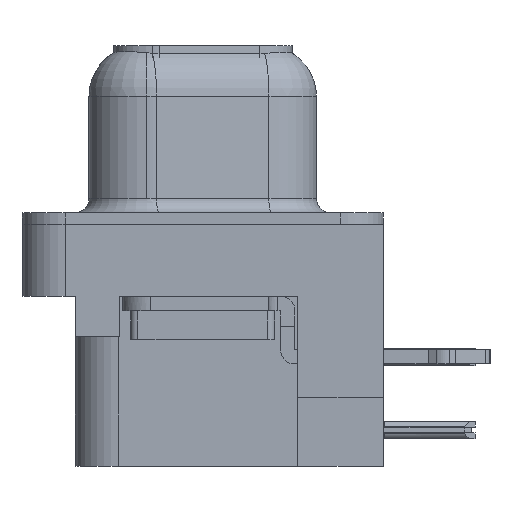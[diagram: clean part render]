
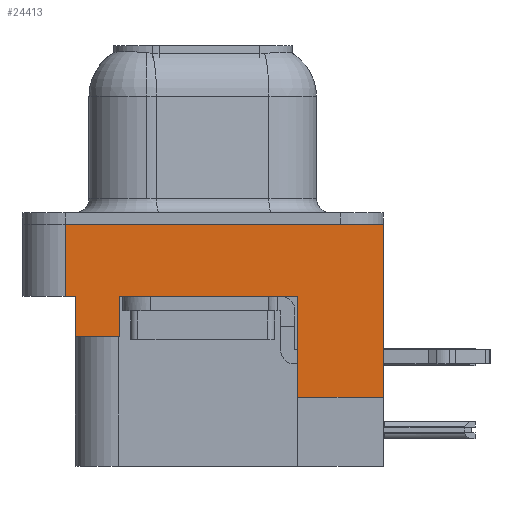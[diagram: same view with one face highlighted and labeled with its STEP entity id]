
A CAD part, left-side view. The second image highlights one B-rep face of the part: STEP entity #24413.
In plain terms, the highlighted planar face has unit normal (-1, 0, 0).
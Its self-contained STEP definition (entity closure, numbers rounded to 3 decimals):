
#319 = LINE ( 'NONE', #17291, #12870 ) ;
#1310 = ORIENTED_EDGE ( 'NONE', *, *, #6165, .T. ) ;
#1367 = LINE ( 'NONE', #1907, #23469 ) ;
#1438 = ORIENTED_EDGE ( 'NONE', *, *, #18184, .F. ) ;
#1659 = LINE ( 'NONE', #19444, #14207 ) ;
#1801 = FACE_OUTER_BOUND ( 'NONE', #29616, .T. ) ;
#1907 = CARTESIAN_POINT ( 'NONE',  ( -3., -6.275, -2.5 ) ) ;
#2087 = VECTOR ( 'NONE', #20687, 1000. ) ;
#2411 = ORIENTED_EDGE ( 'NONE', *, *, #9568, .F. ) ;
#2848 = EDGE_CURVE ( 'NONE', #6711, #3648, #4608, .T. ) ;
#3450 = CARTESIAN_POINT ( 'NONE',  ( -3., 4.425, -3.9 ) ) ;
#3648 = VERTEX_POINT ( 'NONE', #15304 ) ;
#4140 = DIRECTION ( 'NONE',  ( 0., -1., 0. ) ) ;
#4244 = VERTEX_POINT ( 'NONE', #17488 ) ;
#4608 = LINE ( 'NONE', #22447, #10203 ) ;
#4682 = ORIENTED_EDGE ( 'NONE', *, *, #6703, .F. ) ;
#4753 = LINE ( 'NONE', #3450, #29193 ) ;
#5299 = DIRECTION ( 'NONE',  ( 0., 0., 1. ) ) ;
#6165 = EDGE_CURVE ( 'NONE', #25804, #26135, #6997, .T. ) ;
#6294 = ORIENTED_EDGE ( 'NONE', *, *, #2848, .F. ) ;
#6349 = VERTEX_POINT ( 'NONE', #28585 ) ;
#6559 = CARTESIAN_POINT ( 'NONE',  ( -3., -6.275, -2.5 ) ) ;
#6613 = PLANE ( 'NONE',  #25018 ) ;
#6703 = EDGE_CURVE ( 'NONE', #14418, #26135, #4753, .T. ) ;
#6711 = VERTEX_POINT ( 'NONE', #18254 ) ;
#6811 = VECTOR ( 'NONE', #29866, 1000. ) ;
#6997 = LINE ( 'NONE', #28722, #17396 ) ;
#7016 = CARTESIAN_POINT ( 'NONE',  ( -3., -6.275, 0. ) ) ;
#7042 = ORIENTED_EDGE ( 'NONE', *, *, #26446, .F. ) ;
#7494 = CARTESIAN_POINT ( 'NONE',  ( -3., 4.425, -3.9 ) ) ;
#8110 = CARTESIAN_POINT ( 'NONE',  ( -3., 2.895, -3.9 ) ) ;
#8123 = VERTEX_POINT ( 'NONE', #22096 ) ;
#8321 = LINE ( 'NONE', #13397, #6811 ) ;
#8331 = LINE ( 'NONE', #6559, #2087 ) ;
#9023 = DIRECTION ( 'NONE',  ( 0., 0., 1. ) ) ;
#9568 = EDGE_CURVE ( 'NONE', #4244, #13794, #319, .T. ) ;
#10203 = VECTOR ( 'NONE', #22515, 1000. ) ;
#10426 = EDGE_CURVE ( 'NONE', #6711, #13794, #8331, .T. ) ;
#11331 = LINE ( 'NONE', #18085, #23062 ) ;
#11769 = EDGE_CURVE ( 'NONE', #3648, #8123, #1659, .T. ) ;
#12002 = ORIENTED_EDGE ( 'NONE', *, *, #10426, .T. ) ;
#12870 = VECTOR ( 'NONE', #19626, 1000. ) ;
#13397 = CARTESIAN_POINT ( 'NONE',  ( -3., 2.895, -3.9 ) ) ;
#13794 = VERTEX_POINT ( 'NONE', #7016 ) ;
#14207 = VECTOR ( 'NONE', #5299, 1000. ) ;
#14418 = VERTEX_POINT ( 'NONE', #7494 ) ;
#15006 = CARTESIAN_POINT ( 'NONE',  ( -3., 4.425, -2.5 ) ) ;
#15304 = CARTESIAN_POINT ( 'NONE',  ( -3., -3.295, -6. ) ) ;
#15512 = DIRECTION ( 'NONE',  ( 0., 0., 1. ) ) ;
#15846 = CARTESIAN_POINT ( 'NONE',  ( -3., -6.275, -2.5 ) ) ;
#17291 = CARTESIAN_POINT ( 'NONE',  ( -3., -6.275, 0. ) ) ;
#17396 = VECTOR ( 'NONE', #22102, 1000. ) ;
#17465 = ORIENTED_EDGE ( 'NONE', *, *, #29282, .T. ) ;
#17488 = CARTESIAN_POINT ( 'NONE',  ( -3., 4.775, 0. ) ) ;
#18085 = CARTESIAN_POINT ( 'NONE',  ( -3., 4.775, -2.5 ) ) ;
#18184 = EDGE_CURVE ( 'NONE', #25804, #4244, #11331, .T. ) ;
#18254 = CARTESIAN_POINT ( 'NONE',  ( -3., -6.275, -6. ) ) ;
#19444 = CARTESIAN_POINT ( 'NONE',  ( -3., -3.295, -8.4 ) ) ;
#19626 = DIRECTION ( 'NONE',  ( 0., -1., 0. ) ) ;
#20409 = DIRECTION ( 'NONE',  ( 0., 0., 1. ) ) ;
#20687 = DIRECTION ( 'NONE',  ( 0., 0., 1. ) ) ;
#21362 = VECTOR ( 'NONE', #27892, 1000. ) ;
#22096 = CARTESIAN_POINT ( 'NONE',  ( -3., -3.295, -2.5 ) ) ;
#22102 = DIRECTION ( 'NONE',  ( 0., -1., 0. ) ) ;
#22447 = CARTESIAN_POINT ( 'NONE',  ( -3., -6.495, -6. ) ) ;
#22515 = DIRECTION ( 'NONE',  ( 0., 1., 0. ) ) ;
#23062 = VECTOR ( 'NONE', #20409, 1000. ) ;
#23132 = DIRECTION ( 'NONE',  ( -1., 0., 0. ) ) ;
#23469 = VECTOR ( 'NONE', #4140, 1000. ) ;
#23614 = VERTEX_POINT ( 'NONE', #8110 ) ;
#24413 = ADVANCED_FACE ( 'NONE', ( #1801 ), #6613, .T. ) ;
#25018 = AXIS2_PLACEMENT_3D ( 'NONE', #15846, #23132, #9023 ) ;
#25510 = CARTESIAN_POINT ( 'NONE',  ( -3., 4.425, -3.9 ) ) ;
#25804 = VERTEX_POINT ( 'NONE', #28026 ) ;
#26135 = VERTEX_POINT ( 'NONE', #15006 ) ;
#26446 = EDGE_CURVE ( 'NONE', #23614, #14418, #28419, .T. ) ;
#27892 = DIRECTION ( 'NONE',  ( 0., 1., 0. ) ) ;
#27959 = ORIENTED_EDGE ( 'NONE', *, *, #11769, .F. ) ;
#28026 = CARTESIAN_POINT ( 'NONE',  ( -3., 4.775, -2.5 ) ) ;
#28419 = LINE ( 'NONE', #25510, #21362 ) ;
#28585 = CARTESIAN_POINT ( 'NONE',  ( -3., 2.895, -2.5 ) ) ;
#28722 = CARTESIAN_POINT ( 'NONE',  ( -3., -6.275, -2.5 ) ) ;
#29184 = EDGE_CURVE ( 'NONE', #23614, #6349, #8321, .T. ) ;
#29193 = VECTOR ( 'NONE', #15512, 1000. ) ;
#29282 = EDGE_CURVE ( 'NONE', #6349, #8123, #1367, .T. ) ;
#29616 = EDGE_LOOP ( 'NONE', ( #6294, #12002, #2411, #1438, #1310, #4682, #7042, #29679, #17465, #27959 ) ) ;
#29679 = ORIENTED_EDGE ( 'NONE', *, *, #29184, .T. ) ;
#29866 = DIRECTION ( 'NONE',  ( 0., 0., 1. ) ) ;
